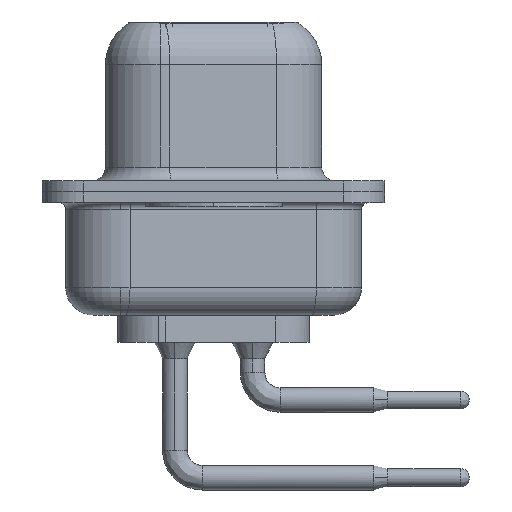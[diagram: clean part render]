
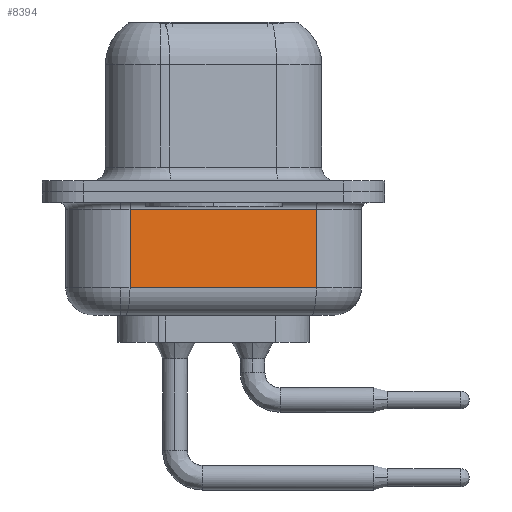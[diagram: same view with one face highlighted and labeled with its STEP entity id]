
A CAD part, left-side view. The second image highlights one B-rep face of the part: STEP entity #8394.
In plain terms, the highlighted planar face has unit normal (-0.985, -0.174, 0).
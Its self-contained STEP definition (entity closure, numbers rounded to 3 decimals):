
#532 = VERTEX_POINT ( 'NONE', #9276 ) ;
#1073 = VECTOR ( 'NONE', #4733, 1000. ) ;
#1226 = EDGE_CURVE ( 'NONE', #4516, #3911, #15613, .T. ) ;
#2050 = ORIENTED_EDGE ( 'NONE', *, *, #1226, .F. ) ;
#2436 = FACE_OUTER_BOUND ( 'NONE', #12519, .T. ) ;
#2533 = VERTEX_POINT ( 'NONE', #3051 ) ;
#3051 = CARTESIAN_POINT ( 'NONE',  ( 4.079, -3.747, -3.5 ) ) ;
#3646 = EDGE_CURVE ( 'NONE', #4516, #2533, #4904, .T. ) ;
#3702 = DIRECTION ( 'NONE',  ( 0., 0., 1. ) ) ;
#3911 = VERTEX_POINT ( 'NONE', #12044 ) ;
#4516 = VERTEX_POINT ( 'NONE', #13500 ) ;
#4733 = DIRECTION ( 'NONE',  ( -0.174, 0.985, 0. ) ) ;
#4764 = CARTESIAN_POINT ( 'NONE',  ( 2.88, 3.053, -0.65 ) ) ;
#4867 = DIRECTION ( 'NONE',  ( -0.174, 0.985, 0. ) ) ;
#4904 = LINE ( 'NONE', #12480, #7853 ) ;
#4928 = DIRECTION ( 'NONE',  ( 0.985, 0.174, 0. ) ) ;
#4989 = PLANE ( 'NONE',  #9279 ) ;
#5197 = CARTESIAN_POINT ( 'NONE',  ( 2.88, 3.053, -4.5 ) ) ;
#5573 = LINE ( 'NONE', #4764, #1073 ) ;
#7667 = EDGE_CURVE ( 'NONE', #532, #3911, #5573, .T. ) ;
#7853 = VECTOR ( 'NONE', #13994, 1000. ) ;
#8204 = LINE ( 'NONE', #15667, #11168 ) ;
#8251 = DIRECTION ( 'NONE',  ( 0., 0., 1. ) ) ;
#8394 = ADVANCED_FACE ( 'NONE', ( #2436 ), #4989, .F. ) ;
#9276 = CARTESIAN_POINT ( 'NONE',  ( 4.079, -3.747, -0.65 ) ) ;
#9279 = AXIS2_PLACEMENT_3D ( 'NONE', #5197, #4928, #4867 ) ;
#10470 = ORIENTED_EDGE ( 'NONE', *, *, #7667, .T. ) ;
#11168 = VECTOR ( 'NONE', #8251, 1000. ) ;
#12044 = CARTESIAN_POINT ( 'NONE',  ( 2.88, 3.053, -0.65 ) ) ;
#12435 = VECTOR ( 'NONE', #3702, 1000. ) ;
#12480 = CARTESIAN_POINT ( 'NONE',  ( 2.88, 3.053, -3.5 ) ) ;
#12519 = EDGE_LOOP ( 'NONE', ( #2050, #14394, #13057, #10470 ) ) ;
#13057 = ORIENTED_EDGE ( 'NONE', *, *, #13910, .T. ) ;
#13500 = CARTESIAN_POINT ( 'NONE',  ( 2.88, 3.053, -3.5 ) ) ;
#13910 = EDGE_CURVE ( 'NONE', #2533, #532, #8204, .T. ) ;
#13994 = DIRECTION ( 'NONE',  ( 0.174, -0.985, 0. ) ) ;
#14250 = CARTESIAN_POINT ( 'NONE',  ( 2.88, 3.053, -4.5 ) ) ;
#14394 = ORIENTED_EDGE ( 'NONE', *, *, #3646, .T. ) ;
#15613 = LINE ( 'NONE', #14250, #12435 ) ;
#15667 = CARTESIAN_POINT ( 'NONE',  ( 4.079, -3.747, -4.5 ) ) ;
